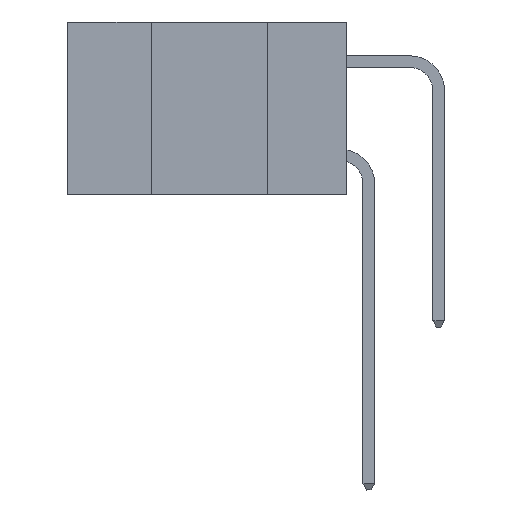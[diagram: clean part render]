
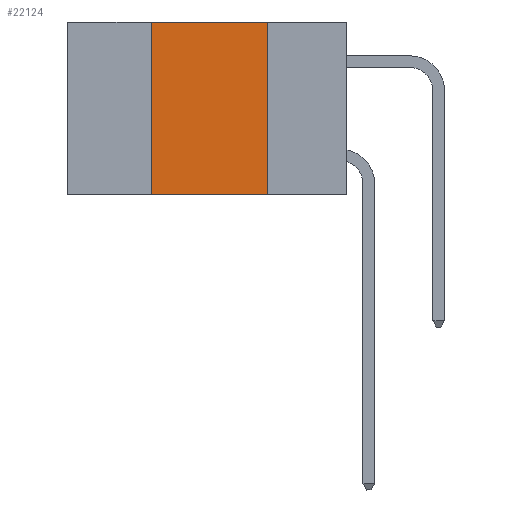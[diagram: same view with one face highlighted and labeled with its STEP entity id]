
A CAD part, left-side view. The second image highlights one B-rep face of the part: STEP entity #22124.
In plain terms, the highlighted planar face has unit normal (-1, 0, 0).
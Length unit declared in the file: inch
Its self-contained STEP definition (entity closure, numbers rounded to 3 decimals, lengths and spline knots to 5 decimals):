
#516 = ORIENTED_EDGE ( 'NONE', *, *, #10527, .F. ) ;
#940 = VERTEX_POINT ( 'NONE', #7509 ) ;
#1660 = CARTESIAN_POINT ( 'NONE',  ( 0., 0.6, 0. ) ) ;
#1698 = VECTOR ( 'NONE', #14264, 39.37008 ) ;
#2314 = LINE ( 'NONE', #12403, #1698 ) ;
#3195 = DIRECTION ( 'NONE',  ( 0., -1., 0. ) ) ;
#3862 = EDGE_CURVE ( 'NONE', #20483, #940, #10228, .T. ) ;
#4364 = VERTEX_POINT ( 'NONE', #19213 ) ;
#4825 = FACE_OUTER_BOUND ( 'NONE', #15641, .T. ) ;
#5086 = VECTOR ( 'NONE', #13082, 39.37008 ) ;
#5707 = EDGE_CURVE ( 'NONE', #20483, #4364, #10144, .T. ) ;
#7509 = CARTESIAN_POINT ( 'NONE',  ( 0., 0.17, -0.37 ) ) ;
#7567 = DIRECTION ( 'NONE',  ( 0., -1., 0. ) ) ;
#7769 = CARTESIAN_POINT ( 'NONE',  ( 0., 0.42, -0.37 ) ) ;
#7839 = CARTESIAN_POINT ( 'NONE',  ( 0., 0.17, 0. ) ) ;
#9200 = CARTESIAN_POINT ( 'NONE',  ( 0., 0.6, 0. ) ) ;
#10144 = LINE ( 'NONE', #18485, #5086 ) ;
#10228 = LINE ( 'NONE', #11175, #19407 ) ;
#10527 = EDGE_CURVE ( 'NONE', #4364, #21075, #20313, .T. ) ;
#11048 = DIRECTION ( 'NONE',  ( 0., 0., -1. ) ) ;
#11136 = VECTOR ( 'NONE', #7567, 39.37008 ) ;
#11175 = CARTESIAN_POINT ( 'NONE',  ( 0., 0.6, -0.37 ) ) ;
#11464 = ORIENTED_EDGE ( 'NONE', *, *, #5707, .F. ) ;
#12050 = ORIENTED_EDGE ( 'NONE', *, *, #3862, .T. ) ;
#12403 = CARTESIAN_POINT ( 'NONE',  ( 0., 0.17, 0. ) ) ;
#13082 = DIRECTION ( 'NONE',  ( 0., 0., 1. ) ) ;
#14264 = DIRECTION ( 'NONE',  ( 0., 0., -1. ) ) ;
#14681 = PLANE ( 'NONE',  #20543 ) ;
#15641 = EDGE_LOOP ( 'NONE', ( #20069, #516, #11464, #12050 ) ) ;
#18485 = CARTESIAN_POINT ( 'NONE',  ( 0., 0.42, 0. ) ) ;
#19213 = CARTESIAN_POINT ( 'NONE',  ( 0., 0.42, 0. ) ) ;
#19407 = VECTOR ( 'NONE', #3195, 39.37008 ) ;
#20069 = ORIENTED_EDGE ( 'NONE', *, *, #21368, .F. ) ;
#20313 = LINE ( 'NONE', #1660, #11136 ) ;
#20483 = VERTEX_POINT ( 'NONE', #7769 ) ;
#20543 = AXIS2_PLACEMENT_3D ( 'NONE', #9200, #21996, #11048 ) ;
#21075 = VERTEX_POINT ( 'NONE', #7839 ) ;
#21368 = EDGE_CURVE ( 'NONE', #21075, #940, #2314, .T. ) ;
#21996 = DIRECTION ( 'NONE',  ( 1., 0., 0. ) ) ;
#22124 = ADVANCED_FACE ( 'NONE', ( #4825 ), #14681, .F. ) ;
